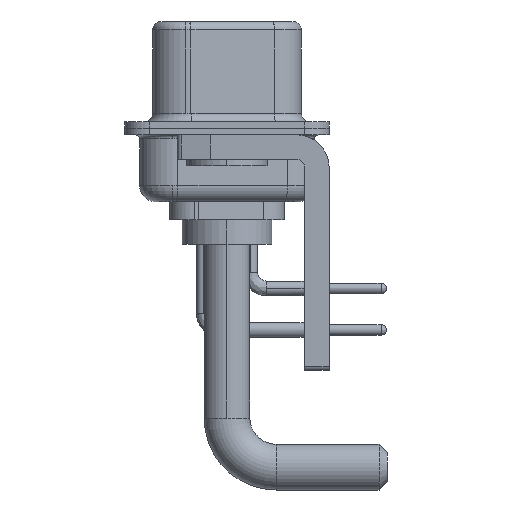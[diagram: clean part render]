
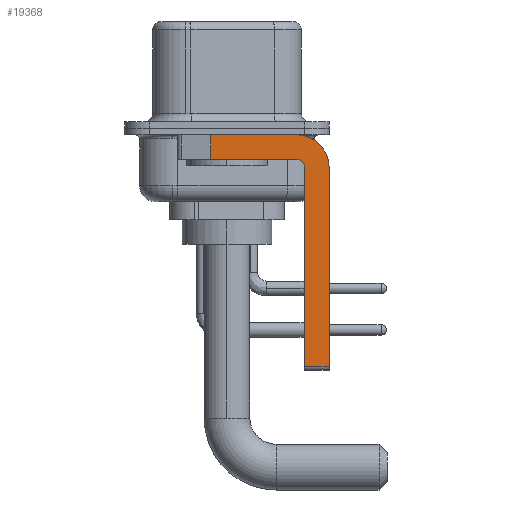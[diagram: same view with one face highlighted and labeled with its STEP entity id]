
A CAD part, left-side view. The second image highlights one B-rep face of the part: STEP entity #19368.
In plain terms, the highlighted planar face has unit normal (-1, 0, 0).
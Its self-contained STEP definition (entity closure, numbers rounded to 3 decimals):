
#127 = DIRECTION ( 'NONE',  ( 0., 0., -1. ) ) ;
#343 = ORIENTED_EDGE ( 'NONE', *, *, #9681, .F. ) ;
#703 = EDGE_CURVE ( 'NONE', #19428, #11038, #9070, .T. ) ;
#2371 = DIRECTION ( 'NONE',  ( 0., 0., 1. ) ) ;
#2459 = ORIENTED_EDGE ( 'NONE', *, *, #703, .F. ) ;
#4133 = VECTOR ( 'NONE', #22697, 1000. ) ;
#4583 = FACE_OUTER_BOUND ( 'NONE', #15731, .T. ) ;
#5360 = DIRECTION ( 'NONE',  ( 0., 1., 0. ) ) ;
#5397 = VERTEX_POINT ( 'NONE', #15311 ) ;
#5469 = DIRECTION ( 'NONE',  ( 0., 0., 1. ) ) ;
#5647 = VECTOR ( 'NONE', #24516, 1000. ) ;
#5655 = DIRECTION ( 'NONE',  ( 1., 0., 0. ) ) ;
#5658 = LINE ( 'NONE', #9933, #17145 ) ;
#6974 = VERTEX_POINT ( 'NONE', #13013 ) ;
#7010 = AXIS2_PLACEMENT_3D ( 'NONE', #16918, #5655, #10234 ) ;
#7104 = CARTESIAN_POINT ( 'NONE',  ( -2.9, -4.75, -14.8 ) ) ;
#7532 = LINE ( 'NONE', #27982, #9018 ) ;
#7726 = VERTEX_POINT ( 'NONE', #10416 ) ;
#9018 = VECTOR ( 'NONE', #25773, 1000. ) ;
#9070 = LINE ( 'NONE', #22280, #5647 ) ;
#9288 = CARTESIAN_POINT ( 'NONE',  ( -2.9, -6.25, -14.55 ) ) ;
#9573 = VECTOR ( 'NONE', #14925, 1000. ) ;
#9677 = ORIENTED_EDGE ( 'NONE', *, *, #18407, .F. ) ;
#9681 = EDGE_CURVE ( 'NONE', #21362, #19428, #28326, .T. ) ;
#9933 = CARTESIAN_POINT ( 'NONE',  ( -2.9, -4.25, -1.9 ) ) ;
#10234 = DIRECTION ( 'NONE',  ( 0., 0., -1. ) ) ;
#10248 = LINE ( 'NONE', #22551, #4133 ) ;
#10416 = CARTESIAN_POINT ( 'NONE',  ( -2.9, 0.978, -1.9 ) ) ;
#10663 = EDGE_CURVE ( 'NONE', #6974, #5397, #17957, .T. ) ;
#10815 = AXIS2_PLACEMENT_3D ( 'NONE', #16426, #12119, #5469 ) ;
#10956 = CARTESIAN_POINT ( 'NONE',  ( -2.9, -6.25, -2.4 ) ) ;
#11038 = VERTEX_POINT ( 'NONE', #9288 ) ;
#11342 = EDGE_CURVE ( 'NONE', #11662, #7726, #21898, .T. ) ;
#11662 = VERTEX_POINT ( 'NONE', #23489 ) ;
#12119 = DIRECTION ( 'NONE',  ( -1., 0., 0. ) ) ;
#12550 = CARTESIAN_POINT ( 'NONE',  ( -2.9, 0.978, -1.9 ) ) ;
#13013 = CARTESIAN_POINT ( 'NONE',  ( -2.9, -4.75, -14.55 ) ) ;
#14925 = DIRECTION ( 'NONE',  ( 0., 0., -1. ) ) ;
#15311 = CARTESIAN_POINT ( 'NONE',  ( -2.9, -4.75, -2.4 ) ) ;
#15731 = EDGE_LOOP ( 'NONE', ( #9677, #22169, #24032, #25014, #23879, #18641, #2459, #343 ) ) ;
#15990 = CARTESIAN_POINT ( 'NONE',  ( -2.9, -4.25, -2.4 ) ) ;
#16426 = CARTESIAN_POINT ( 'NONE',  ( -2.9, -4.25, -2.4 ) ) ;
#16918 = CARTESIAN_POINT ( 'NONE',  ( -2.9, -4.25, -2.4 ) ) ;
#17145 = VECTOR ( 'NONE', #5360, 1000. ) ;
#17957 = LINE ( 'NONE', #7104, #26489 ) ;
#18220 = CARTESIAN_POINT ( 'NONE',  ( -2.9, -4.25, -0.4 ) ) ;
#18407 = EDGE_CURVE ( 'NONE', #11662, #21362, #10248, .T. ) ;
#18641 = ORIENTED_EDGE ( 'NONE', *, *, #25501, .T. ) ;
#19368 = ADVANCED_FACE ( 'NONE', ( #4583 ), #20442, .F. ) ;
#19428 = VERTEX_POINT ( 'NONE', #10956 ) ;
#19541 = EDGE_CURVE ( 'NONE', #5397, #29125, #21258, .T. ) ;
#20442 = PLANE ( 'NONE',  #24549 ) ;
#21258 = CIRCLE ( 'NONE', #10815, 0.5 ) ;
#21362 = VERTEX_POINT ( 'NONE', #18220 ) ;
#21898 = LINE ( 'NONE', #12550, #9573 ) ;
#21923 = CARTESIAN_POINT ( 'NONE',  ( -2.9, -4.25, -1.9 ) ) ;
#22169 = ORIENTED_EDGE ( 'NONE', *, *, #11342, .T. ) ;
#22280 = CARTESIAN_POINT ( 'NONE',  ( -2.9, -6.25, -2.4 ) ) ;
#22551 = CARTESIAN_POINT ( 'NONE',  ( -2.9, 3., -0.4 ) ) ;
#22697 = DIRECTION ( 'NONE',  ( 0., -1., 0. ) ) ;
#23489 = CARTESIAN_POINT ( 'NONE',  ( -2.9, 0.978, -0.4 ) ) ;
#23879 = ORIENTED_EDGE ( 'NONE', *, *, #10663, .F. ) ;
#24032 = ORIENTED_EDGE ( 'NONE', *, *, #26488, .F. ) ;
#24516 = DIRECTION ( 'NONE',  ( 0., 0., -1. ) ) ;
#24549 = AXIS2_PLACEMENT_3D ( 'NONE', #15990, #26675, #127 ) ;
#25014 = ORIENTED_EDGE ( 'NONE', *, *, #19541, .F. ) ;
#25501 = EDGE_CURVE ( 'NONE', #6974, #11038, #7532, .T. ) ;
#25773 = DIRECTION ( 'NONE',  ( 0., -1., 0. ) ) ;
#26488 = EDGE_CURVE ( 'NONE', #29125, #7726, #5658, .T. ) ;
#26489 = VECTOR ( 'NONE', #2371, 1000. ) ;
#26675 = DIRECTION ( 'NONE',  ( 1., 0., 0. ) ) ;
#27982 = CARTESIAN_POINT ( 'NONE',  ( -2.9, -4.25, -14.55 ) ) ;
#28326 = CIRCLE ( 'NONE', #7010, 2. ) ;
#29125 = VERTEX_POINT ( 'NONE', #21923 ) ;
